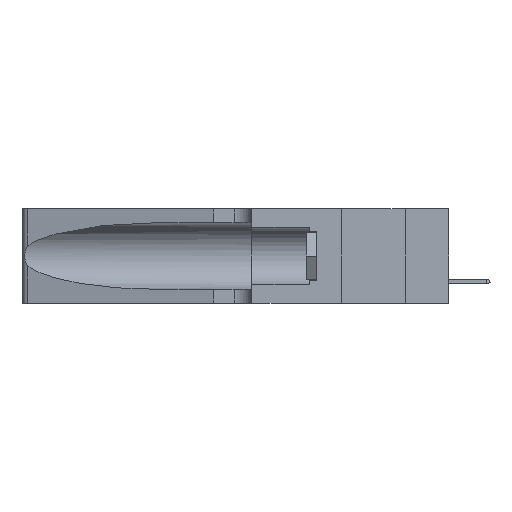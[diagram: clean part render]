
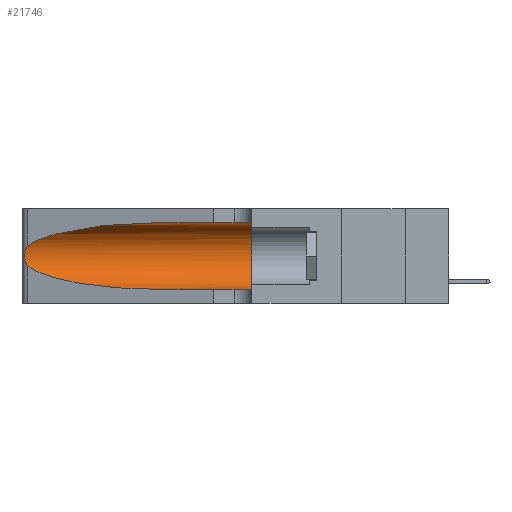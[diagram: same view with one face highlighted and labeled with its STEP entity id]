
A CAD part, left-side view. The second image highlights one B-rep face of the part: STEP entity #21746.
In plain terms, the highlighted cylindrical face has radius 3.308 mm (diameter 6.617 mm), a partial arc.
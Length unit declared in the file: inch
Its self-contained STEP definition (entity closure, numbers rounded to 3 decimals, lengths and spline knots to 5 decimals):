
#615 = CARTESIAN_POINT ( 'NONE',  ( 0.1305, 0.35, 0.31525 ) ) ;
#2249 = EDGE_CURVE ( 'NONE', #8183, #15117, #20519, .T. ) ;
#2263 = LINE ( 'NONE', #13420, #3504 ) ;
#2440 = EDGE_CURVE ( 'NONE', #10404, #13284, #3859, .T. ) ;
#3293 = DIRECTION ( 'NONE',  ( 0., 1., 0. ) ) ;
#3370 = CARTESIAN_POINT ( 'NONE',  ( 0.25787, 1.23484, 0.2124 ) ) ;
#3504 = VECTOR ( 'NONE', #11704, 39.37008 ) ;
#3859 = B_SPLINE_CURVE_WITH_KNOTS ( 'NONE', 3,
 ( #19405, #5493, #19231, #3370, #19157, #25014, #7593, #23154, #11431, #15387, #23236, #7848, #6070, #3939 ),
 .UNSPECIFIED., .F., .F.,
 ( 4, 2, 2, 2, 2, 2, 4 ),
 ( 0., 0.00027, 0.00053, 0.00107, 0.0016, 0.00187, 0.00214 ),
 .UNSPECIFIED. ) ;
#3939 = CARTESIAN_POINT ( 'NONE',  ( 0.25487, 1.22718, 0.14631 ) ) ;
#4692 = CARTESIAN_POINT ( 'NONE',  ( 0.1305, 0.35, 0.05475 ) ) ;
#4823 = DIRECTION ( 'NONE',  ( 0., 0., 1. ) ) ;
#5493 = CARTESIAN_POINT ( 'NONE',  ( 0.25555, 1.22994, 0.2215 ) ) ;
#5498 = CYLINDRICAL_SURFACE ( 'NONE', #16919, 0.13025 ) ;
#5866 = ORIENTED_EDGE ( 'NONE', *, *, #12969, .F. ) ;
#6058 = EDGE_CURVE ( 'NONE', #16167, #10404, #16012, .T. ) ;
#6070 = CARTESIAN_POINT ( 'NONE',  ( 0.25555, 1.22993, 0.14849 ) ) ;
#6086 = DIRECTION ( 'NONE',  ( 0., -1., 0. ) ) ;
#6093 = DIRECTION ( 'NONE',  ( 0., -1., 0. ) ) ;
#6483 = CARTESIAN_POINT ( 'NONE',  ( 0.18966, 0.96281, 0.05475 ) ) ;
#6524 = ORIENTED_EDGE ( 'NONE', *, *, #20967, .T. ) ;
#6678 = CARTESIAN_POINT ( 'NONE',  ( 0.1305, 0.72297, 0.31525 ) ) ;
#7593 = CARTESIAN_POINT ( 'NONE',  ( 0.26075, 1.23896, 0.19203 ) ) ;
#7848 = CARTESIAN_POINT ( 'NONE',  ( 0.25639, 1.23186, 0.15144 ) ) ;
#7851 = CARTESIAN_POINT ( 'NONE',  ( 0.18966, 0.96281, 0.31525 ) ) ;
#8183 = VERTEX_POINT ( 'NONE', #615 ) ;
#8763 = CARTESIAN_POINT ( 'NONE',  ( 0.2373, 1.15595, 0.08982 ) ) ;
#9145 = CARTESIAN_POINT ( 'NONE',  ( 0.1305, 0.35, 0.185 ) ) ;
#10404 = VERTEX_POINT ( 'NONE', #14122 ) ;
#10840 = CARTESIAN_POINT ( 'NONE',  ( 0.1305, 0.72297, 0.05475 ) ) ;
#10866 = EDGE_CURVE ( 'NONE', #13284, #13552, #12537, .T. ) ;
#11431 = CARTESIAN_POINT ( 'NONE',  ( 0.26017, 1.23833, 0.17102 ) ) ;
#11704 = DIRECTION ( 'NONE',  ( 0., -1., 0. ) ) ;
#11772 = CARTESIAN_POINT ( 'NONE',  ( 0.25487, 1.22718, 0.22369 ) ) ;
#12537 =( BOUNDED_CURVE ( )  B_SPLINE_CURVE ( 3, ( #17803, #8763, #6483, #10840 ),
 .UNSPECIFIED., .F., .T. ) 
 B_SPLINE_CURVE_WITH_KNOTS ( ( 4, 4 ),
 ( 3.44316, 4.71239 ),
 .UNSPECIFIED. ) 
 CURVE ( )  GEOMETRIC_REPRESENTATION_ITEM ( )  RATIONAL_B_SPLINE_CURVE ( ( 1., 0.87, 0.87, 1. ) ) 
 REPRESENTATION_ITEM ( '' )  );
#12969 = EDGE_CURVE ( 'NONE', #16167, #8183, #2263, .T. ) ;
#13284 = VERTEX_POINT ( 'NONE', #23908 ) ;
#13420 = CARTESIAN_POINT ( 'NONE',  ( 0.1305, 1.61858, 0.31525 ) ) ;
#13552 = VERTEX_POINT ( 'NONE', #18693 ) ;
#14122 = CARTESIAN_POINT ( 'NONE',  ( 0.25487, 1.22718, 0.22369 ) ) ;
#15117 = VERTEX_POINT ( 'NONE', #4692 ) ;
#15387 = CARTESIAN_POINT ( 'NONE',  ( 0.25856, 1.23593, 0.16098 ) ) ;
#15401 = VECTOR ( 'NONE', #6093, 39.37008 ) ;
#15997 = CARTESIAN_POINT ( 'NONE',  ( 0.1305, 1.61858, 0.185 ) ) ;
#16012 =( BOUNDED_CURVE ( )  B_SPLINE_CURVE ( 3, ( #23574, #7851, #21532, #11772 ),
 .UNSPECIFIED., .F., .F. ) 
 B_SPLINE_CURVE_WITH_KNOTS ( ( 4, 4 ),
 ( 1.5708, 2.84003 ),
 .UNSPECIFIED. ) 
 CURVE ( )  GEOMETRIC_REPRESENTATION_ITEM ( )  RATIONAL_B_SPLINE_CURVE ( ( 1., 0.87, 0.87, 1. ) ) 
 REPRESENTATION_ITEM ( '' )  );
#16167 = VERTEX_POINT ( 'NONE', #6678 ) ;
#16919 = AXIS2_PLACEMENT_3D ( 'NONE', #15997, #6086, #19755 ) ;
#17690 = CARTESIAN_POINT ( 'NONE',  ( 0.1305, 1.61858, 0.05475 ) ) ;
#17803 = CARTESIAN_POINT ( 'NONE',  ( 0.25487, 1.22718, 0.14631 ) ) ;
#18071 = FACE_OUTER_BOUND ( 'NONE', #19625, .T. ) ;
#18693 = CARTESIAN_POINT ( 'NONE',  ( 0.1305, 0.72297, 0.05475 ) ) ;
#18936 = ORIENTED_EDGE ( 'NONE', *, *, #10866, .T. ) ;
#19157 = CARTESIAN_POINT ( 'NONE',  ( 0.25854, 1.2359, 0.20912 ) ) ;
#19231 = CARTESIAN_POINT ( 'NONE',  ( 0.25639, 1.23184, 0.21858 ) ) ;
#19405 = CARTESIAN_POINT ( 'NONE',  ( 0.25487, 1.22718, 0.22369 ) ) ;
#19625 = EDGE_LOOP ( 'NONE', ( #23927, #24469, #18936, #6524, #20591, #5866 ) ) ;
#19755 = DIRECTION ( 'NONE',  ( 0., 0., -1. ) ) ;
#20289 = LINE ( 'NONE', #17690, #15401 ) ;
#20519 = CIRCLE ( 'NONE', #24672, 0.13025 ) ;
#20591 = ORIENTED_EDGE ( 'NONE', *, *, #2249, .F. ) ;
#20967 = EDGE_CURVE ( 'NONE', #13552, #15117, #20289, .T. ) ;
#21532 = CARTESIAN_POINT ( 'NONE',  ( 0.2373, 1.15595, 0.28018 ) ) ;
#21746 = ADVANCED_FACE ( 'NONE', ( #18071 ), #5498, .F. ) ;
#23154 = CARTESIAN_POINT ( 'NONE',  ( 0.26075, 1.23896, 0.178 ) ) ;
#23236 = CARTESIAN_POINT ( 'NONE',  ( 0.25789, 1.23486, 0.15765 ) ) ;
#23574 = CARTESIAN_POINT ( 'NONE',  ( 0.1305, 0.72297, 0.31525 ) ) ;
#23908 = CARTESIAN_POINT ( 'NONE',  ( 0.25487, 1.22718, 0.14631 ) ) ;
#23927 = ORIENTED_EDGE ( 'NONE', *, *, #6058, .T. ) ;
#24469 = ORIENTED_EDGE ( 'NONE', *, *, #2440, .T. ) ;
#24672 = AXIS2_PLACEMENT_3D ( 'NONE', #9145, #3293, #4823 ) ;
#25014 = CARTESIAN_POINT ( 'NONE',  ( 0.26018, 1.23835, 0.19895 ) ) ;
